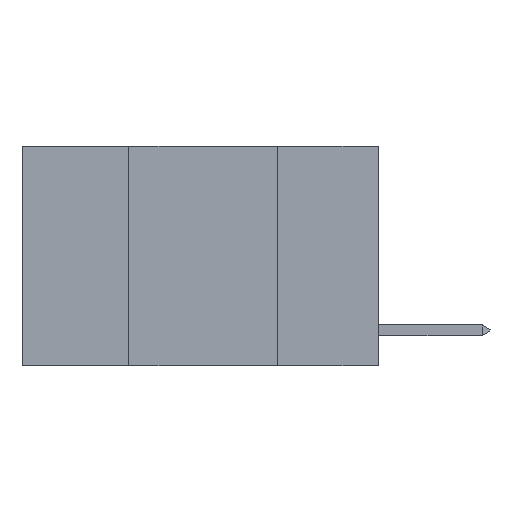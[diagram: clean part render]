
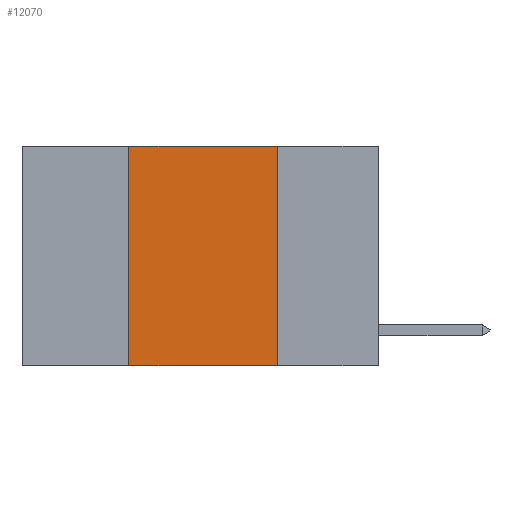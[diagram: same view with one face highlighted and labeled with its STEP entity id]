
A CAD part, left-side view. The second image highlights one B-rep face of the part: STEP entity #12070.
In plain terms, the highlighted planar face has unit normal (-1, 0, 0).
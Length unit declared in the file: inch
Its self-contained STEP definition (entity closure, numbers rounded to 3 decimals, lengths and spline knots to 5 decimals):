
#1026 = VECTOR ( 'NONE', #22246, 39.37008 ) ;
#1537 = LINE ( 'NONE', #14775, #1026 ) ;
#2835 = ORIENTED_EDGE ( 'NONE', *, *, #16372, .F. ) ;
#3258 = LINE ( 'NONE', #10707, #21624 ) ;
#3498 = VECTOR ( 'NONE', #11739, 39.37008 ) ;
#3914 = CARTESIAN_POINT ( 'NONE',  ( 0., 0.6, 0. ) ) ;
#4100 = ORIENTED_EDGE ( 'NONE', *, *, #19575, .F. ) ;
#4162 = LINE ( 'NONE', #3914, #3498 ) ;
#4939 = EDGE_LOOP ( 'NONE', ( #12506, #4100, #2835, #19305 ) ) ;
#5057 = DIRECTION ( 'NONE',  ( 0., 0., 1. ) ) ;
#5202 = CARTESIAN_POINT ( 'NONE',  ( 0., 0.17, 0. ) ) ;
#6111 = AXIS2_PLACEMENT_3D ( 'NONE', #20327, #14532, #16639 ) ;
#6666 = CARTESIAN_POINT ( 'NONE',  ( 0., 0.42, -0.37 ) ) ;
#6903 = EDGE_CURVE ( 'NONE', #12311, #17806, #3258, .T. ) ;
#10707 = CARTESIAN_POINT ( 'NONE',  ( 0., 0.6, -0.37 ) ) ;
#11739 = DIRECTION ( 'NONE',  ( 0., -1., 0. ) ) ;
#11761 = VECTOR ( 'NONE', #5057, 39.37008 ) ;
#12070 = ADVANCED_FACE ( 'NONE', ( #18226 ), #12721, .F. ) ;
#12311 = VERTEX_POINT ( 'NONE', #6666 ) ;
#12506 = ORIENTED_EDGE ( 'NONE', *, *, #15882, .F. ) ;
#12721 = PLANE ( 'NONE',  #6111 ) ;
#13484 = CARTESIAN_POINT ( 'NONE',  ( 0., 0.17, -0.37 ) ) ;
#13912 = CARTESIAN_POINT ( 'NONE',  ( 0., 0.42, 0. ) ) ;
#14501 = DIRECTION ( 'NONE',  ( 0., -1., 0. ) ) ;
#14532 = DIRECTION ( 'NONE',  ( 1., 0., 0. ) ) ;
#14775 = CARTESIAN_POINT ( 'NONE',  ( 0., 0.17, 0. ) ) ;
#15712 = VERTEX_POINT ( 'NONE', #13912 ) ;
#15882 = EDGE_CURVE ( 'NONE', #17625, #17806, #1537, .T. ) ;
#16372 = EDGE_CURVE ( 'NONE', #12311, #15712, #16681, .T. ) ;
#16639 = DIRECTION ( 'NONE',  ( 0., 0., -1. ) ) ;
#16681 = LINE ( 'NONE', #23807, #11761 ) ;
#17625 = VERTEX_POINT ( 'NONE', #5202 ) ;
#17806 = VERTEX_POINT ( 'NONE', #13484 ) ;
#18226 = FACE_OUTER_BOUND ( 'NONE', #4939, .T. ) ;
#19305 = ORIENTED_EDGE ( 'NONE', *, *, #6903, .T. ) ;
#19575 = EDGE_CURVE ( 'NONE', #15712, #17625, #4162, .T. ) ;
#20327 = CARTESIAN_POINT ( 'NONE',  ( 0., 0.6, 0. ) ) ;
#21624 = VECTOR ( 'NONE', #14501, 39.37008 ) ;
#22246 = DIRECTION ( 'NONE',  ( 0., 0., -1. ) ) ;
#23807 = CARTESIAN_POINT ( 'NONE',  ( 0., 0.42, 0. ) ) ;
